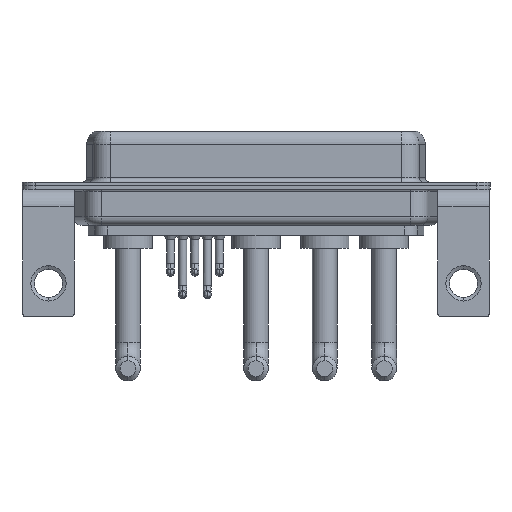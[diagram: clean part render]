
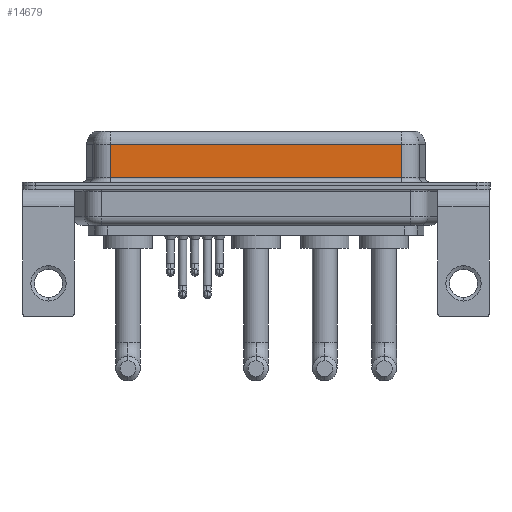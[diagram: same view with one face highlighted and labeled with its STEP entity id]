
A CAD part, front view. The second image highlights one B-rep face of the part: STEP entity #14679.
In plain terms, the highlighted planar face has unit normal (0, -1, 0).
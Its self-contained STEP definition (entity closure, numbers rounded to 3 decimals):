
#1872 = LINE ( 'NONE', #17292, #5871 ) ;
#2051 = DIRECTION ( 'NONE',  ( 0., 0., -1. ) ) ;
#3037 = ORIENTED_EDGE ( 'NONE', *, *, #4126, .F. ) ;
#3069 = VERTEX_POINT ( 'NONE', #7031 ) ;
#3338 = EDGE_LOOP ( 'NONE', ( #3037, #11500, #7845, #13391 ) ) ;
#3418 = EDGE_CURVE ( 'NONE', #3069, #15834, #5609, .T. ) ;
#3499 = DIRECTION ( 'NONE',  ( 0., 0., -1. ) ) ;
#4126 = EDGE_CURVE ( 'NONE', #15277, #15834, #14002, .T. ) ;
#5609 = LINE ( 'NONE', #8440, #5921 ) ;
#5871 = VECTOR ( 'NONE', #2051, 1000. ) ;
#5921 = VECTOR ( 'NONE', #16667, 1000. ) ;
#7031 = CARTESIAN_POINT ( 'NONE',  ( 7.013, -3.95, 0.9 ) ) ;
#7208 = EDGE_CURVE ( 'NONE', #15277, #16548, #11329, .T. ) ;
#7845 = ORIENTED_EDGE ( 'NONE', *, *, #17240, .T. ) ;
#8418 = AXIS2_PLACEMENT_3D ( 'NONE', #16875, #15687, #11490 ) ;
#8440 = CARTESIAN_POINT ( 'NONE',  ( 40.037, -3.95, 0.9 ) ) ;
#9449 = VECTOR ( 'NONE', #15524, 1000. ) ;
#9959 = CARTESIAN_POINT ( 'NONE',  ( 40.037, -3.95, 4.65 ) ) ;
#11329 = LINE ( 'NONE', #9959, #9449 ) ;
#11490 = DIRECTION ( 'NONE',  ( 0., 0., 1. ) ) ;
#11500 = ORIENTED_EDGE ( 'NONE', *, *, #7208, .T. ) ;
#11923 = CARTESIAN_POINT ( 'NONE',  ( 7.013, -3.95, 4.65 ) ) ;
#12628 = CARTESIAN_POINT ( 'NONE',  ( 40.037, -3.95, 4.65 ) ) ;
#12772 = FACE_OUTER_BOUND ( 'NONE', #3338, .T. ) ;
#13391 = ORIENTED_EDGE ( 'NONE', *, *, #3418, .T. ) ;
#14002 = LINE ( 'NONE', #14535, #15584 ) ;
#14404 = PLANE ( 'NONE',  #8418 ) ;
#14535 = CARTESIAN_POINT ( 'NONE',  ( 40.037, -3.95, 6.4 ) ) ;
#14679 = ADVANCED_FACE ( 'NONE', ( #12772 ), #14404, .F. ) ;
#15277 = VERTEX_POINT ( 'NONE', #12628 ) ;
#15524 = DIRECTION ( 'NONE',  ( -1., 0., 0. ) ) ;
#15584 = VECTOR ( 'NONE', #3499, 1000. ) ;
#15687 = DIRECTION ( 'NONE',  ( 0., 1., 0. ) ) ;
#15700 = CARTESIAN_POINT ( 'NONE',  ( 40.037, -3.95, 0.9 ) ) ;
#15834 = VERTEX_POINT ( 'NONE', #15700 ) ;
#16548 = VERTEX_POINT ( 'NONE', #11923 ) ;
#16667 = DIRECTION ( 'NONE',  ( 1., 0., 0. ) ) ;
#16875 = CARTESIAN_POINT ( 'NONE',  ( 40.037, -3.95, 6.4 ) ) ;
#17240 = EDGE_CURVE ( 'NONE', #16548, #3069, #1872, .T. ) ;
#17292 = CARTESIAN_POINT ( 'NONE',  ( 7.013, -3.95, 6.4 ) ) ;
